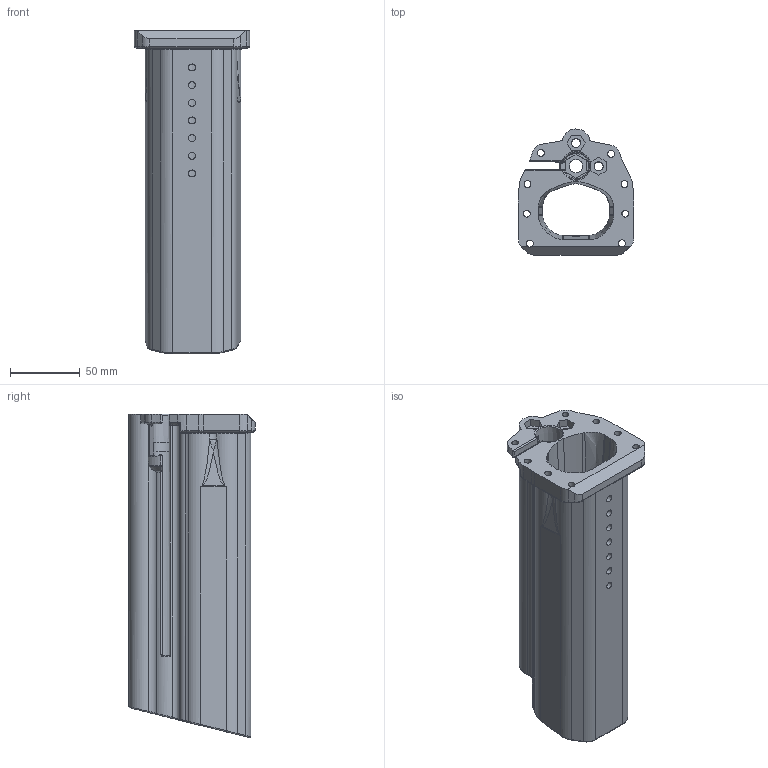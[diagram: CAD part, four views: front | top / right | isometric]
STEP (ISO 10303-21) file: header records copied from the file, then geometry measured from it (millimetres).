
FILE_DESCRIPTION(/* description */ ('STEP AP214'),/* implementation_level */ '2;1');
FILE_NAME(/* name */ 'PSG-style handguard-default catch-type2.stp',/* time_stamp */ '2021-11-25T00:07:11-06:00',/* author */ ('johne'),/* organization */ (''),/* preprocessor_version */ 'ST-DEVELOPER v18.1',/* originating_system */ 'Autodesk Inventor 2020',/* authorisation */ '');
FILE_SCHEMA (('AUTOMOTIVE_DESIGN { 1 0 10303 214 3 1 1 }'));
Length unit declared in the file: inch
Products named in the file (1): PSG-style handguard- default catch
Bounding box: 82.76 x 90.63 x 232.45 mm (x, y, z)
Volume: 528397.4 mm3; surface area: 121977.5 mm2
Topology: 1 solids, 1 shells, 370 faces, 995 edges, 611 vertices
Faces by surface type: cylinder 127, bspline 117, plane 73, torus 40, cone 8, sphere 5
Full cylindrical faces by diameter (mm): 5 x15, 6.477 x2, 9.525 x1
Entity records: 16287 total; most frequent: CARTESIAN_POINT 7514, ORIENTED_EDGE 1958, DIRECTION 1679, EDGE_CURVE 979, AXIS2_PLACEMENT_3D 667, VERTEX_POINT 611, EDGE_LOOP 408, FACE_OUTER_BOUND 370
